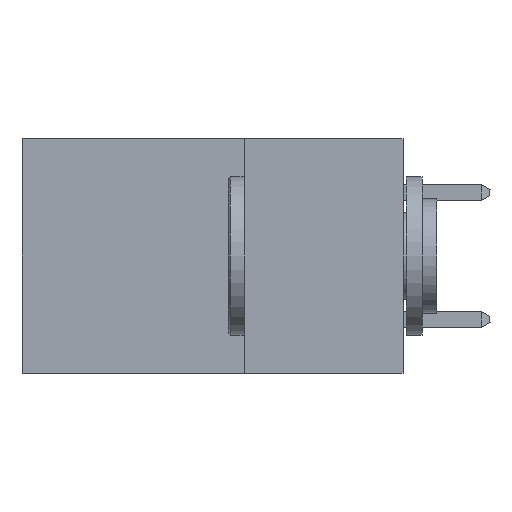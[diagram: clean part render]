
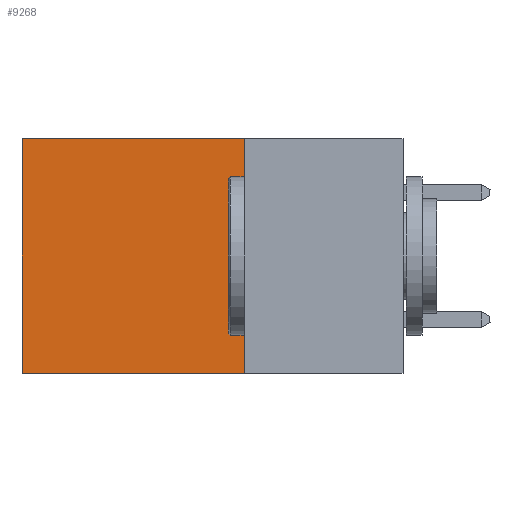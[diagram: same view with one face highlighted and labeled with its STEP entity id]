
A CAD part, left-side view. The second image highlights one B-rep face of the part: STEP entity #9268.
In plain terms, the highlighted planar face has unit normal (-1, 0, 0).
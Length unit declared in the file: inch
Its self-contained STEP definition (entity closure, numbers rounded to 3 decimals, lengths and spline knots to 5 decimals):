
#47 = EDGE_CURVE ( 'NONE', #8164, #2578, #1927, .T. ) ;
#552 = DIRECTION ( 'NONE',  ( 0., 0., -1. ) ) ;
#1016 = EDGE_LOOP ( 'NONE', ( #1152, #3011, #2144, #7523 ) ) ;
#1152 = ORIENTED_EDGE ( 'NONE', *, *, #3395, .T. ) ;
#1434 = VECTOR ( 'NONE', #6000, 39.37008 ) ;
#1819 = LINE ( 'NONE', #9704, #4203 ) ;
#1927 = LINE ( 'NONE', #2562, #1434 ) ;
#2144 = ORIENTED_EDGE ( 'NONE', *, *, #47, .F. ) ;
#2562 = CARTESIAN_POINT ( 'NONE',  ( 0.2875, 0.25, 0. ) ) ;
#2578 = VERTEX_POINT ( 'NONE', #4544 ) ;
#2729 = DIRECTION ( 'NONE',  ( 0., 0., -1. ) ) ;
#2881 = CARTESIAN_POINT ( 'NONE',  ( 0.2875, 0.25, 0. ) ) ;
#3011 = ORIENTED_EDGE ( 'NONE', *, *, #4738, .F. ) ;
#3395 = EDGE_CURVE ( 'NONE', #4386, #4685, #8064, .T. ) ;
#4203 = VECTOR ( 'NONE', #9718, 39.37008 ) ;
#4386 = VERTEX_POINT ( 'NONE', #7950 ) ;
#4415 = EDGE_CURVE ( 'NONE', #8164, #4386, #7037, .T. ) ;
#4482 = PLANE ( 'NONE',  #6754 ) ;
#4544 = CARTESIAN_POINT ( 'NONE',  ( 0.2875, 0.25, -0.37 ) ) ;
#4685 = VERTEX_POINT ( 'NONE', #8854 ) ;
#4728 = CARTESIAN_POINT ( 'NONE',  ( 0.2875, 0.25, 0. ) ) ;
#4738 = EDGE_CURVE ( 'NONE', #2578, #4685, #1819, .T. ) ;
#4833 = VECTOR ( 'NONE', #10019, 39.37008 ) ;
#5321 = DIRECTION ( 'NONE',  ( 1., 0., 0. ) ) ;
#5645 = FACE_OUTER_BOUND ( 'NONE', #1016, .T. ) ;
#6000 = DIRECTION ( 'NONE',  ( 0., 0., -1. ) ) ;
#6754 = AXIS2_PLACEMENT_3D ( 'NONE', #2881, #5321, #552 ) ;
#7037 = LINE ( 'NONE', #8608, #4833 ) ;
#7523 = ORIENTED_EDGE ( 'NONE', *, *, #4415, .T. ) ;
#7817 = VECTOR ( 'NONE', #2729, 39.37008 ) ;
#7950 = CARTESIAN_POINT ( 'NONE',  ( 0.2875, 0.6, 0. ) ) ;
#8064 = LINE ( 'NONE', #10107, #7817 ) ;
#8164 = VERTEX_POINT ( 'NONE', #4728 ) ;
#8608 = CARTESIAN_POINT ( 'NONE',  ( 0.2875, 0.25, 0. ) ) ;
#8854 = CARTESIAN_POINT ( 'NONE',  ( 0.2875, 0.6, -0.37 ) ) ;
#9268 = ADVANCED_FACE ( 'NONE', ( #5645 ), #4482, .F. ) ;
#9704 = CARTESIAN_POINT ( 'NONE',  ( 0.2875, 0.25, -0.37 ) ) ;
#9718 = DIRECTION ( 'NONE',  ( 0., 1., 0. ) ) ;
#10019 = DIRECTION ( 'NONE',  ( 0., 1., 0. ) ) ;
#10107 = CARTESIAN_POINT ( 'NONE',  ( 0.2875, 0.6, 0. ) ) ;
